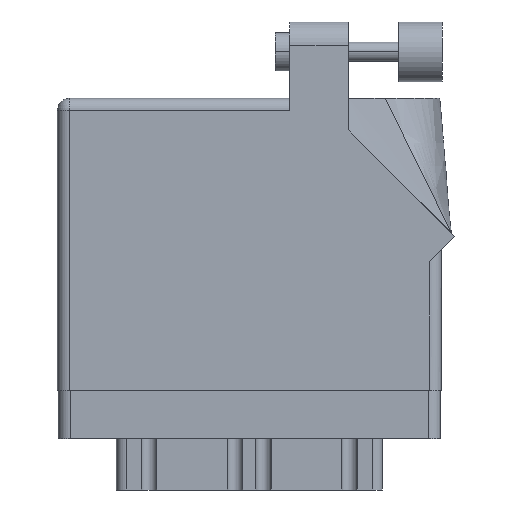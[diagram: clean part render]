
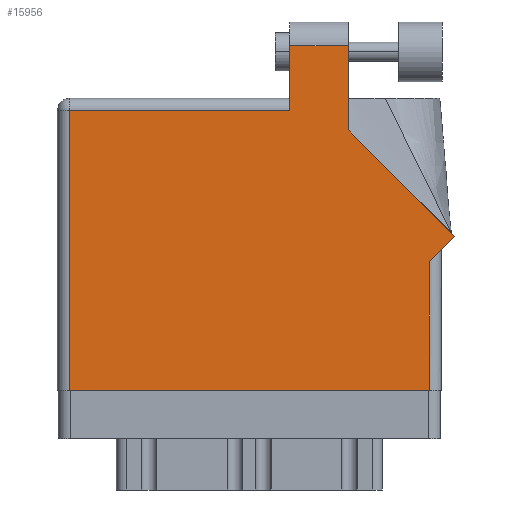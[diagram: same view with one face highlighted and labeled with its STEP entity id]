
A CAD part, front view. The second image highlights one B-rep face of the part: STEP entity #15956.
In plain terms, the highlighted face is planar.
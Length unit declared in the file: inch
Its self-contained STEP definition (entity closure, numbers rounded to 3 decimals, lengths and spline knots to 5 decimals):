
#1083 = DIRECTION ( 'NONE',  ( -1., 0., 0. ) ) ;
#1282 = VERTEX_POINT ( 'NONE', #17455 ) ;
#1419 = LINE ( 'NONE', #24327, #22843 ) ;
#1565 = ORIENTED_EDGE ( 'NONE', *, *, #5054, .T. ) ;
#3541 = VECTOR ( 'NONE', #31597, 39.37008 ) ;
#5054 = EDGE_CURVE ( 'NONE', #1282, #20030, #20414, .T. ) ;
#6587 = VECTOR ( 'NONE', #22778, 39.37008 ) ;
#6634 = VERTEX_POINT ( 'NONE', #16101 ) ;
#6935 = ORIENTED_EDGE ( 'NONE', *, *, #20830, .T. ) ;
#7435 = DIRECTION ( 'NONE',  ( 0., 1., 0. ) ) ;
#7526 = CARTESIAN_POINT ( 'NONE',  ( 1.948, 0., 0. ) ) ;
#7710 = LINE ( 'NONE', #19644, #3541 ) ;
#7820 = EDGE_LOOP ( 'NONE', ( #13865, #30656, #1565, #30871, #11753, #19280, #8008, #23023, #6935 ) ) ;
#8008 = ORIENTED_EDGE ( 'NONE', *, *, #24158, .T. ) ;
#8270 = LINE ( 'NONE', #20398, #37658 ) ;
#8988 = CARTESIAN_POINT ( 'NONE',  ( 1.524, 1.36442, 0. ) ) ;
#10280 = FACE_OUTER_BOUND ( 'NONE', #7820, .T. ) ;
#10748 = DIRECTION ( 'NONE',  ( -0.707, 0.707, 0. ) ) ;
#10846 = CARTESIAN_POINT ( 'NONE',  ( 1.217, 1.53, 0. ) ) ;
#11158 = CARTESIAN_POINT ( 'NONE',  ( 1.948, 0.737, 0. ) ) ;
#11345 = CARTESIAN_POINT ( 'NONE',  ( 0., 0., 0. ) ) ;
#11753 = ORIENTED_EDGE ( 'NONE', *, *, #18928, .T. ) ;
#11931 = VERTEX_POINT ( 'NONE', #18366 ) ;
#13613 = DIRECTION ( 'NONE',  ( 0., 0., -1. ) ) ;
#13865 = ORIENTED_EDGE ( 'NONE', *, *, #33100, .T. ) ;
#14532 = EDGE_CURVE ( 'NONE', #31594, #11931, #1419, .T. ) ;
#15544 = VERTEX_POINT ( 'NONE', #31664 ) ;
#15627 = EDGE_CURVE ( 'NONE', #20030, #34826, #26348, .T. ) ;
#15952 = CARTESIAN_POINT ( 'NONE',  ( 0., 1.53, 0. ) ) ;
#15956 = ADVANCED_FACE ( 'NONE', ( #10280 ), #22210, .F. ) ;
#16101 = CARTESIAN_POINT ( 'NONE',  ( 0.062, 0., 0. ) ) ;
#16752 = VERTEX_POINT ( 'NONE', #33287 ) ;
#17055 = EDGE_CURVE ( 'NONE', #6634, #38643, #35424, .T. ) ;
#17455 = CARTESIAN_POINT ( 'NONE',  ( 1.217, 1.805, 0. ) ) ;
#17593 = DIRECTION ( 'NONE',  ( 1., 0., 0. ) ) ;
#17613 = DIRECTION ( 'NONE',  ( 0., 1., 0. ) ) ;
#18037 = AXIS2_PLACEMENT_3D ( 'NONE', #15952, #13613, #1083 ) ;
#18366 = CARTESIAN_POINT ( 'NONE',  ( 2.08071, 0.80771, 0. ) ) ;
#18928 = EDGE_CURVE ( 'NONE', #34826, #6634, #8270, .T. ) ;
#18992 = VECTOR ( 'NONE', #38709, 39.37008 ) ;
#19280 = ORIENTED_EDGE ( 'NONE', *, *, #17055, .T. ) ;
#19644 = CARTESIAN_POINT ( 'NONE',  ( 1.217, 1.805, 0. ) ) ;
#19724 = CARTESIAN_POINT ( 'NONE',  ( 2.08071, 0.80771, 0. ) ) ;
#19877 = CARTESIAN_POINT ( 'NONE',  ( 1.217, 1.468, 0. ) ) ;
#20030 = VERTEX_POINT ( 'NONE', #19877 ) ;
#20398 = CARTESIAN_POINT ( 'NONE',  ( 0.062, 0., 0. ) ) ;
#20414 = LINE ( 'NONE', #10846, #6587 ) ;
#20830 = EDGE_CURVE ( 'NONE', #11931, #16752, #34440, .T. ) ;
#21204 = VECTOR ( 'NONE', #7435, 39.37008 ) ;
#22210 = PLANE ( 'NONE',  #18037 ) ;
#22505 = CARTESIAN_POINT ( 'NONE',  ( 0.062, 1.468, 0. ) ) ;
#22778 = DIRECTION ( 'NONE',  ( 0., -1., 0. ) ) ;
#22843 = VECTOR ( 'NONE', #27647, 39.37008 ) ;
#23023 = ORIENTED_EDGE ( 'NONE', *, *, #14532, .T. ) ;
#24158 = EDGE_CURVE ( 'NONE', #38643, #31594, #31330, .T. ) ;
#24327 = CARTESIAN_POINT ( 'NONE',  ( 2.01, 0.737, 0. ) ) ;
#26348 = LINE ( 'NONE', #29669, #18992 ) ;
#27647 = DIRECTION ( 'NONE',  ( 0.707, 0.707, 0. ) ) ;
#29022 = DIRECTION ( 'NONE',  ( 0., -1., 0. ) ) ;
#29375 = LINE ( 'NONE', #8988, #33779 ) ;
#29669 = CARTESIAN_POINT ( 'NONE',  ( 0., 1.468, 0. ) ) ;
#30656 = ORIENTED_EDGE ( 'NONE', *, *, #35735, .T. ) ;
#30871 = ORIENTED_EDGE ( 'NONE', *, *, #15627, .T. ) ;
#31330 = LINE ( 'NONE', #11158, #21204 ) ;
#31594 = VERTEX_POINT ( 'NONE', #33584 ) ;
#31597 = DIRECTION ( 'NONE',  ( -1., 0., 0. ) ) ;
#31664 = CARTESIAN_POINT ( 'NONE',  ( 1.524, 1.805, 0. ) ) ;
#33100 = EDGE_CURVE ( 'NONE', #16752, #15544, #29375, .T. ) ;
#33287 = CARTESIAN_POINT ( 'NONE',  ( 1.524, 1.36442, 0. ) ) ;
#33584 = CARTESIAN_POINT ( 'NONE',  ( 1.948, 0.675, 0. ) ) ;
#33779 = VECTOR ( 'NONE', #17613, 39.37008 ) ;
#34440 = LINE ( 'NONE', #19724, #37578 ) ;
#34718 = VECTOR ( 'NONE', #17593, 39.37008 ) ;
#34826 = VERTEX_POINT ( 'NONE', #22505 ) ;
#35424 = LINE ( 'NONE', #11345, #34718 ) ;
#35735 = EDGE_CURVE ( 'NONE', #15544, #1282, #7710, .T. ) ;
#37578 = VECTOR ( 'NONE', #10748, 39.37008 ) ;
#37658 = VECTOR ( 'NONE', #29022, 39.37008 ) ;
#38643 = VERTEX_POINT ( 'NONE', #7526 ) ;
#38709 = DIRECTION ( 'NONE',  ( -1., 0., 0. ) ) ;
